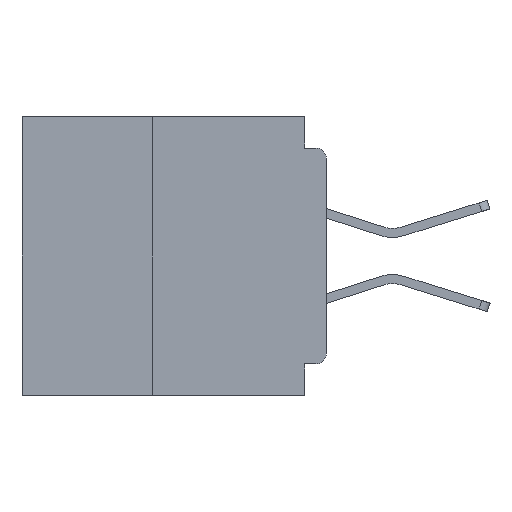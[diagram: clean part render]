
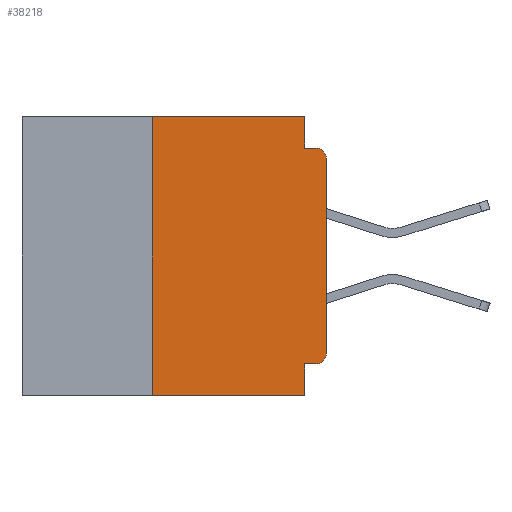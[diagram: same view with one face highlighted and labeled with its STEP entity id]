
A CAD part, left-side view. The second image highlights one B-rep face of the part: STEP entity #38218.
In plain terms, the highlighted planar face has unit normal (-1, 0, 0).
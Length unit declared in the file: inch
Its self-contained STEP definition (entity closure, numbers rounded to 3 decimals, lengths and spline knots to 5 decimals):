
#1483 = CARTESIAN_POINT ( 'NONE',  ( 0., 0.031, -0.4 ) ) ;
#2572 = VERTEX_POINT ( 'NONE', #8033 ) ;
#3109 = VERTEX_POINT ( 'NONE', #23165 ) ;
#3183 = CARTESIAN_POINT ( 'NONE',  ( 0., 0., -0.34 ) ) ;
#5127 = CARTESIAN_POINT ( 'NONE',  ( 0., 0.437, -0.4 ) ) ;
#5392 = ORIENTED_EDGE ( 'NONE', *, *, #36081, .F. ) ;
#6287 = ORIENTED_EDGE ( 'NONE', *, *, #50166, .T. ) ;
#8033 = CARTESIAN_POINT ( 'NONE',  ( 0., 0.25, 0. ) ) ;
#8381 = CARTESIAN_POINT ( 'NONE',  ( 0., 0., 0. ) ) ;
#8868 = CARTESIAN_POINT ( 'NONE',  ( 0., 0.031, -0.4 ) ) ;
#9808 = CARTESIAN_POINT ( 'NONE',  ( 0., 0., -0.06 ) ) ;
#9880 = DIRECTION ( 'NONE',  ( 0., -1., 0. ) ) ;
#10225 = CARTESIAN_POINT ( 'NONE',  ( 0., 0.015, -0.34 ) ) ;
#10404 = CARTESIAN_POINT ( 'NONE',  ( 0., 0., -0.045 ) ) ;
#10513 = EDGE_CURVE ( 'NONE', #3109, #2572, #18594, .T. ) ;
#10626 = VERTEX_POINT ( 'NONE', #14935 ) ;
#11082 = DIRECTION ( 'NONE',  ( 1., 0., 0. ) ) ;
#11969 = EDGE_CURVE ( 'NONE', #12780, #30915, #47042, .T. ) ;
#12597 = EDGE_CURVE ( 'NONE', #43778, #10626, #47690, .T. ) ;
#12780 = VERTEX_POINT ( 'NONE', #15142 ) ;
#14926 = DIRECTION ( 'NONE',  ( 0., 0., -1. ) ) ;
#14935 = CARTESIAN_POINT ( 'NONE',  ( 0., 0.031, -0.355 ) ) ;
#15003 = DIRECTION ( 'NONE',  ( 0., 0., -1. ) ) ;
#15142 = CARTESIAN_POINT ( 'NONE',  ( 0., 0.031, 0. ) ) ;
#16071 = LINE ( 'NONE', #37559, #25731 ) ;
#17902 = DIRECTION ( 'NONE',  ( 0., 0., 1. ) ) ;
#18594 = LINE ( 'NONE', #31957, #40740 ) ;
#18759 = ORIENTED_EDGE ( 'NONE', *, *, #25438, .F. ) ;
#18805 = DIRECTION ( 'NONE',  ( 0., -1., 0. ) ) ;
#20873 = LINE ( 'NONE', #5127, #42943 ) ;
#21003 = DIRECTION ( 'NONE',  ( -1., 0., 0. ) ) ;
#21397 = VECTOR ( 'NONE', #17902, 39.37008 ) ;
#22883 = ORIENTED_EDGE ( 'NONE', *, *, #12597, .F. ) ;
#23116 = DIRECTION ( 'NONE',  ( 0., 0., -1. ) ) ;
#23165 = CARTESIAN_POINT ( 'NONE',  ( 0., 0.25, -0.4 ) ) ;
#24122 = ORIENTED_EDGE ( 'NONE', *, *, #55470, .F. ) ;
#24262 = CIRCLE ( 'NONE', #42469, 0.015 ) ;
#24870 = ORIENTED_EDGE ( 'NONE', *, *, #54717, .T. ) ;
#24930 = ORIENTED_EDGE ( 'NONE', *, *, #10513, .F. ) ;
#25272 = VECTOR ( 'NONE', #23116, 39.37008 ) ;
#25438 = EDGE_CURVE ( 'NONE', #2572, #12780, #16071, .T. ) ;
#25731 = VECTOR ( 'NONE', #18805, 39.37008 ) ;
#26766 = EDGE_CURVE ( 'NONE', #43778, #42570, #58928, .T. ) ;
#27492 = VERTEX_POINT ( 'NONE', #1483 ) ;
#28617 = VERTEX_POINT ( 'NONE', #9808 ) ;
#29441 = DIRECTION ( 'NONE',  ( 0., -1., 0. ) ) ;
#29922 = CARTESIAN_POINT ( 'NONE',  ( 0., 0.015, -0.045 ) ) ;
#30915 = VERTEX_POINT ( 'NONE', #37532 ) ;
#31955 = DIRECTION ( 'NONE',  ( 0., 1., 0. ) ) ;
#31957 = CARTESIAN_POINT ( 'NONE',  ( 0., 0.25, -0.4 ) ) ;
#35317 = VECTOR ( 'NONE', #31955, 39.37008 ) ;
#36081 = EDGE_CURVE ( 'NONE', #10626, #27492, #37755, .T. ) ;
#37532 = CARTESIAN_POINT ( 'NONE',  ( 0., 0.031, -0.045 ) ) ;
#37559 = CARTESIAN_POINT ( 'NONE',  ( 0., 0.437, 0. ) ) ;
#37713 = LINE ( 'NONE', #10404, #48637 ) ;
#37755 = LINE ( 'NONE', #8868, #25272 ) ;
#38218 = ADVANCED_FACE ( 'NONE', ( #50068 ), #43834, .F. ) ;
#40740 = VECTOR ( 'NONE', #50882, 39.37008 ) ;
#42469 = AXIS2_PLACEMENT_3D ( 'NONE', #49071, #21003, #53754 ) ;
#42570 = VERTEX_POINT ( 'NONE', #3183 ) ;
#42943 = VECTOR ( 'NONE', #9880, 39.37008 ) ;
#43180 = DIRECTION ( 'NONE',  ( -1., 0., 0. ) ) ;
#43245 = CARTESIAN_POINT ( 'NONE',  ( 0., 0.031, 0. ) ) ;
#43733 = EDGE_CURVE ( 'NONE', #28617, #51782, #24262, .T. ) ;
#43778 = VERTEX_POINT ( 'NONE', #49266 ) ;
#43834 = PLANE ( 'NONE',  #55075 ) ;
#44031 = DIRECTION ( 'NONE',  ( 0., 0., -1. ) ) ;
#44780 = ORIENTED_EDGE ( 'NONE', *, *, #26766, .T. ) ;
#47042 = LINE ( 'NONE', #43245, #48510 ) ;
#47690 = LINE ( 'NONE', #59776, #35317 ) ;
#48468 = CARTESIAN_POINT ( 'NONE',  ( 0., 0.437, 0. ) ) ;
#48510 = VECTOR ( 'NONE', #15003, 39.37008 ) ;
#48576 = EDGE_LOOP ( 'NONE', ( #6287, #49984, #24122, #58944, #18759, #24930, #24870, #5392, #22883, #44780 ) ) ;
#48637 = VECTOR ( 'NONE', #29441, 39.37008 ) ;
#49071 = CARTESIAN_POINT ( 'NONE',  ( 0., 0.015, -0.06 ) ) ;
#49266 = CARTESIAN_POINT ( 'NONE',  ( 0., 0.015, -0.355 ) ) ;
#49984 = ORIENTED_EDGE ( 'NONE', *, *, #43733, .T. ) ;
#50068 = FACE_OUTER_BOUND ( 'NONE', #48576, .T. ) ;
#50166 = EDGE_CURVE ( 'NONE', #42570, #28617, #58684, .T. ) ;
#50882 = DIRECTION ( 'NONE',  ( 0., 0., 1. ) ) ;
#51782 = VERTEX_POINT ( 'NONE', #29922 ) ;
#52620 = AXIS2_PLACEMENT_3D ( 'NONE', #10225, #43180, #14926 ) ;
#53754 = DIRECTION ( 'NONE',  ( 0., 0., -1. ) ) ;
#54717 = EDGE_CURVE ( 'NONE', #3109, #27492, #20873, .T. ) ;
#55075 = AXIS2_PLACEMENT_3D ( 'NONE', #48468, #11082, #44031 ) ;
#55470 = EDGE_CURVE ( 'NONE', #30915, #51782, #37713, .T. ) ;
#58684 = LINE ( 'NONE', #8381, #21397 ) ;
#58928 = CIRCLE ( 'NONE', #52620, 0.015 ) ;
#58944 = ORIENTED_EDGE ( 'NONE', *, *, #11969, .F. ) ;
#59776 = CARTESIAN_POINT ( 'NONE',  ( 0., 0., -0.355 ) ) ;
